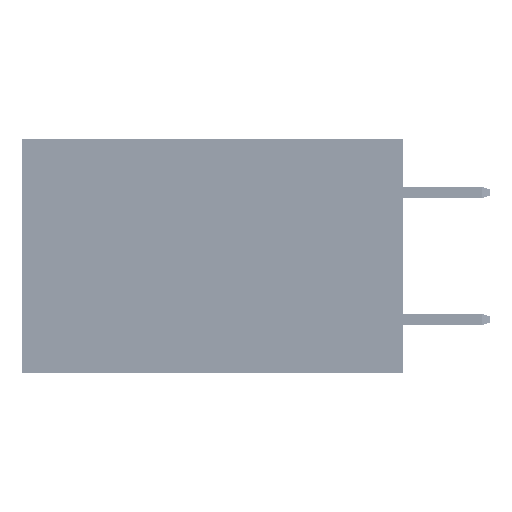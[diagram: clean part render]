
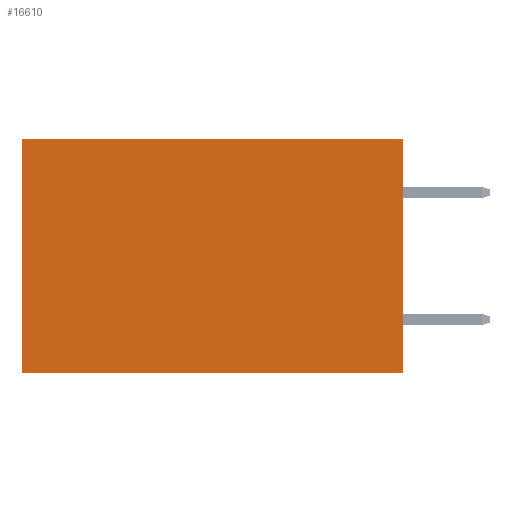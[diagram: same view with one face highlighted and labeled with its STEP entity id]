
A CAD part, left-side view. The second image highlights one B-rep face of the part: STEP entity #16610.
In plain terms, the highlighted planar face has unit normal (-1, 0, 0).
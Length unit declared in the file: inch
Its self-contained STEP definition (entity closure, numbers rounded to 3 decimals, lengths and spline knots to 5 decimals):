
#1431 = CARTESIAN_POINT ( 'NONE',  ( 0.2875, 0., 0. ) ) ;
#1983 = EDGE_CURVE ( 'NONE', #5752, #25802, #14396, .T. ) ;
#2656 = ORIENTED_EDGE ( 'NONE', *, *, #6606, .F. ) ;
#4077 = CARTESIAN_POINT ( 'NONE',  ( 0.2875, 0.6, -0.37 ) ) ;
#4145 = VERTEX_POINT ( 'NONE', #29611 ) ;
#5153 = CARTESIAN_POINT ( 'NONE',  ( 0.2875, 0., 0. ) ) ;
#5247 = AXIS2_PLACEMENT_3D ( 'NONE', #1431, #36376, #9980 ) ;
#5351 = VECTOR ( 'NONE', #20506, 39.37008 ) ;
#5752 = VERTEX_POINT ( 'NONE', #32321 ) ;
#6606 = EDGE_CURVE ( 'NONE', #4145, #42584, #44609, .T. ) ;
#9980 = DIRECTION ( 'NONE',  ( 0., 0., -1. ) ) ;
#11170 = VECTOR ( 'NONE', #41083, 39.37008 ) ;
#13257 = FACE_OUTER_BOUND ( 'NONE', #44556, .T. ) ;
#14396 = LINE ( 'NONE', #22656, #39226 ) ;
#15882 = ORIENTED_EDGE ( 'NONE', *, *, #26497, .F. ) ;
#16610 = ADVANCED_FACE ( 'NONE', ( #13257 ), #28607, .F. ) ;
#18354 = EDGE_CURVE ( 'NONE', #4145, #5752, #39142, .T. ) ;
#20506 = DIRECTION ( 'NONE',  ( 0., 1., 0. ) ) ;
#20616 = CARTESIAN_POINT ( 'NONE',  ( 0.2875, 0., -0.37 ) ) ;
#21637 = CARTESIAN_POINT ( 'NONE',  ( 0.2875, 0., -0.37 ) ) ;
#22656 = CARTESIAN_POINT ( 'NONE',  ( 0.2875, 0.6, 0. ) ) ;
#24922 = ORIENTED_EDGE ( 'NONE', *, *, #1983, .T. ) ;
#25802 = VERTEX_POINT ( 'NONE', #4077 ) ;
#26497 = EDGE_CURVE ( 'NONE', #42584, #25802, #28900, .T. ) ;
#28607 = PLANE ( 'NONE',  #5247 ) ;
#28900 = LINE ( 'NONE', #20616, #35536 ) ;
#29611 = CARTESIAN_POINT ( 'NONE',  ( 0.2875, 0., 0. ) ) ;
#32321 = CARTESIAN_POINT ( 'NONE',  ( 0.2875, 0.6, 0. ) ) ;
#33724 = DIRECTION ( 'NONE',  ( 0., 0., -1. ) ) ;
#34284 = CARTESIAN_POINT ( 'NONE',  ( 0.2875, 0., 0. ) ) ;
#35536 = VECTOR ( 'NONE', #48243, 39.37008 ) ;
#36376 = DIRECTION ( 'NONE',  ( 1., 0., 0. ) ) ;
#39142 = LINE ( 'NONE', #5153, #5351 ) ;
#39226 = VECTOR ( 'NONE', #33724, 39.37008 ) ;
#41083 = DIRECTION ( 'NONE',  ( 0., 0., -1. ) ) ;
#42584 = VERTEX_POINT ( 'NONE', #21637 ) ;
#43376 = ORIENTED_EDGE ( 'NONE', *, *, #18354, .T. ) ;
#44556 = EDGE_LOOP ( 'NONE', ( #24922, #15882, #2656, #43376 ) ) ;
#44609 = LINE ( 'NONE', #34284, #11170 ) ;
#48243 = DIRECTION ( 'NONE',  ( 0., 1., 0. ) ) ;
